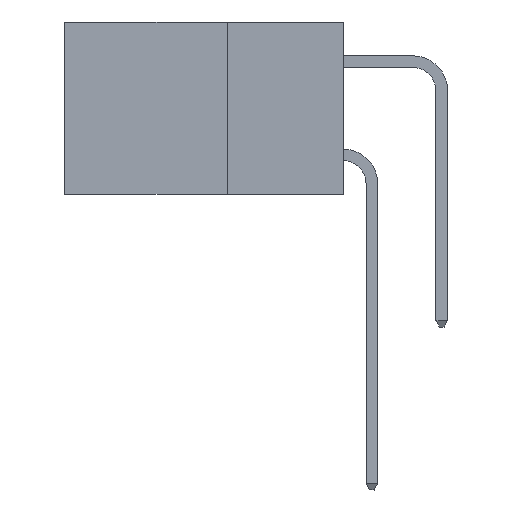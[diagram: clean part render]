
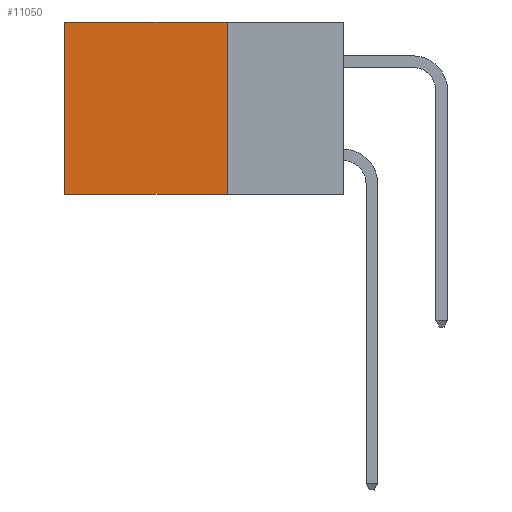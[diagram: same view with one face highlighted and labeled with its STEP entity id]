
A CAD part, left-side view. The second image highlights one B-rep face of the part: STEP entity #11050.
In plain terms, the highlighted planar face has unit normal (-1, 0, 0).
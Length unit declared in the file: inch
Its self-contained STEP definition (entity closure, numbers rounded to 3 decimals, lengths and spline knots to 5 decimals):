
#571 = PLANE ( 'NONE',  #11145 ) ;
#579 = CARTESIAN_POINT ( 'NONE',  ( 0.2615, 0.6, -0.37 ) ) ;
#855 = VECTOR ( 'NONE', #5183, 39.37008 ) ;
#1687 = CARTESIAN_POINT ( 'NONE',  ( 0.2615, 0.25, 0. ) ) ;
#2301 = ORIENTED_EDGE ( 'NONE', *, *, #10714, .T. ) ;
#2501 = VERTEX_POINT ( 'NONE', #5149 ) ;
#2550 = CARTESIAN_POINT ( 'NONE',  ( 0.2615, 0.25, 0. ) ) ;
#2719 = LINE ( 'NONE', #1687, #6695 ) ;
#3105 = LINE ( 'NONE', #6166, #855 ) ;
#4057 = ORIENTED_EDGE ( 'NONE', *, *, #9894, .F. ) ;
#4970 = ORIENTED_EDGE ( 'NONE', *, *, #9720, .F. ) ;
#5149 = CARTESIAN_POINT ( 'NONE',  ( 0.2615, 0.6, 0. ) ) ;
#5183 = DIRECTION ( 'NONE',  ( 0., 0., -1. ) ) ;
#5211 = FACE_OUTER_BOUND ( 'NONE', #6822, .T. ) ;
#5272 = LINE ( 'NONE', #6193, #6282 ) ;
#5578 = CARTESIAN_POINT ( 'NONE',  ( 0.2615, 0.25, -0.37 ) ) ;
#6009 = CARTESIAN_POINT ( 'NONE',  ( 0.2615, 0.25, -0.37 ) ) ;
#6166 = CARTESIAN_POINT ( 'NONE',  ( 0.2615, 0.6, -0.37 ) ) ;
#6193 = CARTESIAN_POINT ( 'NONE',  ( 0.2615, 0.25, -0.37 ) ) ;
#6282 = VECTOR ( 'NONE', #9777, 39.37008 ) ;
#6389 = VERTEX_POINT ( 'NONE', #579 ) ;
#6695 = VECTOR ( 'NONE', #7368, 39.37008 ) ;
#6822 = EDGE_LOOP ( 'NONE', ( #7728, #4057, #4970, #2301 ) ) ;
#6946 = DIRECTION ( 'NONE',  ( 0., 0., -1. ) ) ;
#7177 = DIRECTION ( 'NONE',  ( 1., 0., 0. ) ) ;
#7236 = DIRECTION ( 'NONE',  ( 0., 1., 0. ) ) ;
#7368 = DIRECTION ( 'NONE',  ( 0., 1., 0. ) ) ;
#7728 = ORIENTED_EDGE ( 'NONE', *, *, #11889, .T. ) ;
#7819 = VERTEX_POINT ( 'NONE', #2550 ) ;
#9195 = VECTOR ( 'NONE', #7236, 39.37008 ) ;
#9720 = EDGE_CURVE ( 'NONE', #7819, #11632, #5272, .T. ) ;
#9777 = DIRECTION ( 'NONE',  ( 0., 0., -1. ) ) ;
#9894 = EDGE_CURVE ( 'NONE', #11632, #6389, #10189, .T. ) ;
#10189 = LINE ( 'NONE', #5578, #9195 ) ;
#10714 = EDGE_CURVE ( 'NONE', #7819, #2501, #2719, .T. ) ;
#11050 = ADVANCED_FACE ( 'NONE', ( #5211 ), #571, .F. ) ;
#11145 = AXIS2_PLACEMENT_3D ( 'NONE', #6009, #7177, #6946 ) ;
#11148 = CARTESIAN_POINT ( 'NONE',  ( 0.2615, 0.25, -0.37 ) ) ;
#11632 = VERTEX_POINT ( 'NONE', #11148 ) ;
#11889 = EDGE_CURVE ( 'NONE', #2501, #6389, #3105, .T. ) ;
